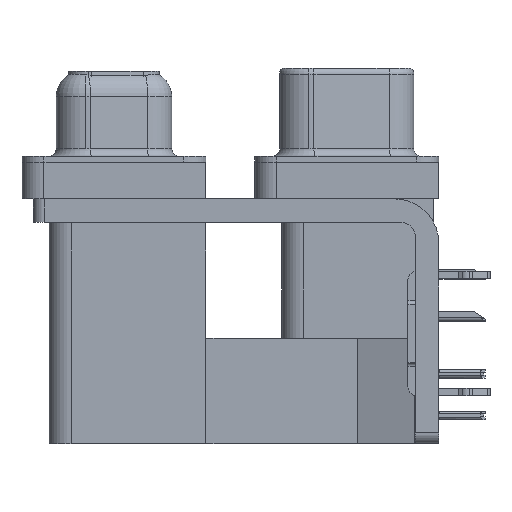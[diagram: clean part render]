
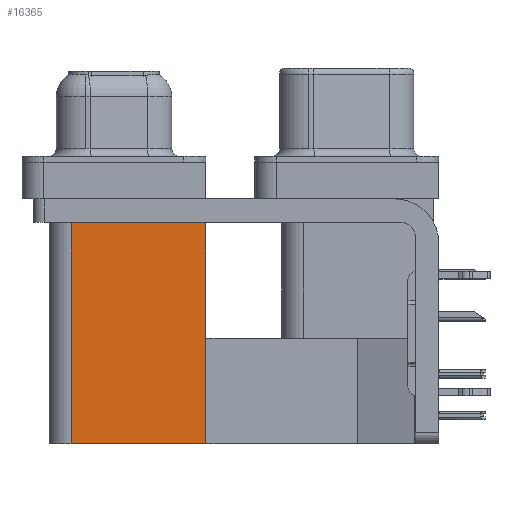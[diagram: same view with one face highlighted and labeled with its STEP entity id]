
A CAD part, left-side view. The second image highlights one B-rep face of the part: STEP entity #16365.
In plain terms, the highlighted planar face has unit normal (-1, 0, 0).
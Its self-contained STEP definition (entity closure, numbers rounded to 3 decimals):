
#47 = CARTESIAN_POINT ( 'NONE',  ( 3.79, 9.6, -19.2 ) ) ;
#223 = CARTESIAN_POINT ( 'NONE',  ( 3.79, 9.6, -19.2 ) ) ;
#564 = EDGE_CURVE ( 'NONE', #13264, #6271, #26847, .T. ) ;
#709 = VERTEX_POINT ( 'NONE', #47 ) ;
#3081 = CARTESIAN_POINT ( 'NONE',  ( 3.79, 9.6, -2.5 ) ) ;
#4476 = LINE ( 'NONE', #26225, #22401 ) ;
#6271 = VERTEX_POINT ( 'NONE', #26360 ) ;
#11093 = CARTESIAN_POINT ( 'NONE',  ( 3.79, 18.8, -19.2 ) ) ;
#13264 = VERTEX_POINT ( 'NONE', #11093 ) ;
#13421 = EDGE_CURVE ( 'NONE', #709, #26995, #4476, .T. ) ;
#14107 = VECTOR ( 'NONE', #32935, 1000. ) ;
#14146 = DIRECTION ( 'NONE',  ( 0., 0., 1. ) ) ;
#14658 = EDGE_CURVE ( 'NONE', #709, #13264, #17226, .T. ) ;
#16365 = ADVANCED_FACE ( 'NONE', ( #21563 ), #27826, .F. ) ;
#17226 = LINE ( 'NONE', #29711, #14107 ) ;
#17369 = EDGE_CURVE ( 'NONE', #26995, #6271, #23866, .T. ) ;
#20379 = VECTOR ( 'NONE', #21007, 1000. ) ;
#21007 = DIRECTION ( 'NONE',  ( 0., 0., 1. ) ) ;
#21563 = FACE_OUTER_BOUND ( 'NONE', #33158, .T. ) ;
#21780 = DIRECTION ( 'NONE',  ( 1., 0., 0. ) ) ;
#21895 = ORIENTED_EDGE ( 'NONE', *, *, #13421, .T. ) ;
#22401 = VECTOR ( 'NONE', #14146, 1000. ) ;
#23866 = LINE ( 'NONE', #39584, #29772 ) ;
#24251 = DIRECTION ( 'NONE',  ( 0., 1., 0. ) ) ;
#24794 = DIRECTION ( 'NONE',  ( 0., 1., 0. ) ) ;
#26225 = CARTESIAN_POINT ( 'NONE',  ( 3.79, 9.6, -19.2 ) ) ;
#26360 = CARTESIAN_POINT ( 'NONE',  ( 3.79, 18.8, -2.5 ) ) ;
#26847 = LINE ( 'NONE', #39357, #20379 ) ;
#26995 = VERTEX_POINT ( 'NONE', #3081 ) ;
#27826 = PLANE ( 'NONE',  #30176 ) ;
#29711 = CARTESIAN_POINT ( 'NONE',  ( 3.79, 9.6, -19.2 ) ) ;
#29772 = VECTOR ( 'NONE', #24251, 1000. ) ;
#30007 = ORIENTED_EDGE ( 'NONE', *, *, #17369, .T. ) ;
#30176 = AXIS2_PLACEMENT_3D ( 'NONE', #223, #21780, #24794 ) ;
#32935 = DIRECTION ( 'NONE',  ( 0., 1., 0. ) ) ;
#33158 = EDGE_LOOP ( 'NONE', ( #30007, #38105, #35448, #21895 ) ) ;
#35448 = ORIENTED_EDGE ( 'NONE', *, *, #14658, .F. ) ;
#38105 = ORIENTED_EDGE ( 'NONE', *, *, #564, .F. ) ;
#39357 = CARTESIAN_POINT ( 'NONE',  ( 3.79, 18.8, -19.2 ) ) ;
#39584 = CARTESIAN_POINT ( 'NONE',  ( 3.79, 9.6, -2.5 ) ) ;
